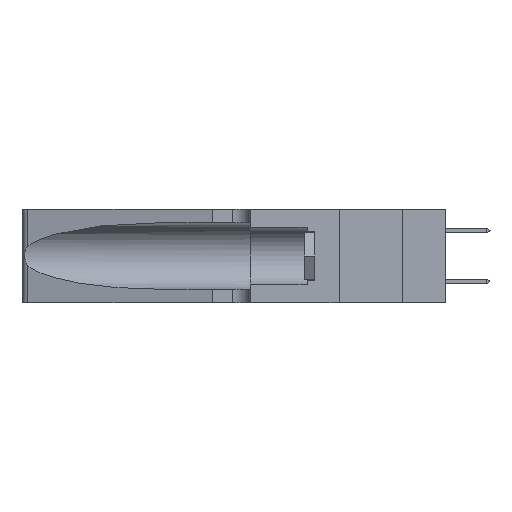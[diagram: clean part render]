
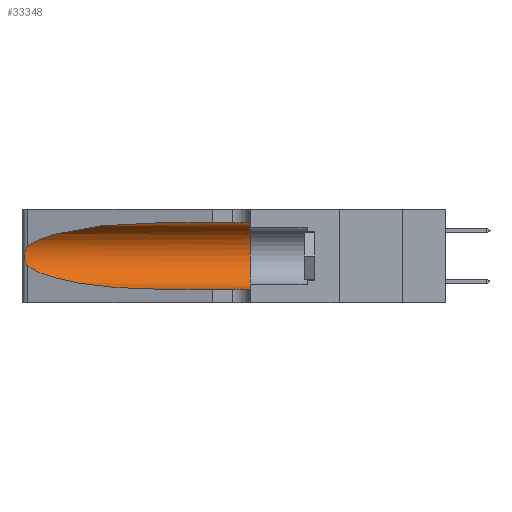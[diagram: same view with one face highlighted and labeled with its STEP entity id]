
A CAD part, left-side view. The second image highlights one B-rep face of the part: STEP entity #33348.
In plain terms, the highlighted cylindrical face has radius 3.308 mm (diameter 6.617 mm), a partial arc.
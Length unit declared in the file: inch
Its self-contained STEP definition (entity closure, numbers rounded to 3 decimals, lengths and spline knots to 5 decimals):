
#203 = FACE_OUTER_BOUND ( 'NONE', #29813, .T. ) ;
#289 = VECTOR ( 'NONE', #3742, 39.37008 ) ;
#589 = CARTESIAN_POINT ( 'NONE',  ( 0.25639, 1.23186, 0.15144 ) ) ;
#987 = EDGE_CURVE ( 'NONE', #16586, #30965, #5221, .T. ) ;
#1922 =( BOUNDED_CURVE ( )  B_SPLINE_CURVE ( 3, ( #33452, #4341, #13200, #30527 ),
 .UNSPECIFIED., .F., .F. ) 
 B_SPLINE_CURVE_WITH_KNOTS ( ( 4, 4 ),
 ( 1.5708, 2.84003 ),
 .UNSPECIFIED. ) 
 CURVE ( )  GEOMETRIC_REPRESENTATION_ITEM ( )  RATIONAL_B_SPLINE_CURVE ( ( 1., 0.87, 0.87, 1. ) ) 
 REPRESENTATION_ITEM ( '' )  );
#2430 = CARTESIAN_POINT ( 'NONE',  ( 0.1305, 0.35, 0.31525 ) ) ;
#3742 = DIRECTION ( 'NONE',  ( 0., -1., 0. ) ) ;
#4259 = CARTESIAN_POINT ( 'NONE',  ( 0.25487, 1.22718, 0.14631 ) ) ;
#4341 = CARTESIAN_POINT ( 'NONE',  ( 0.18966, 0.96281, 0.31525 ) ) ;
#4634 = CARTESIAN_POINT ( 'NONE',  ( 0.18966, 0.96281, 0.05475 ) ) ;
#4980 = ORIENTED_EDGE ( 'NONE', *, *, #33149, .F. ) ;
#5221 =( BOUNDED_CURVE ( )  B_SPLINE_CURVE ( 3, ( #4259, #10405, #4634, #7182 ),
 .UNSPECIFIED., .F., .F. ) 
 B_SPLINE_CURVE_WITH_KNOTS ( ( 4, 4 ),
 ( 3.44316, 4.71239 ),
 .UNSPECIFIED. ) 
 CURVE ( )  GEOMETRIC_REPRESENTATION_ITEM ( )  RATIONAL_B_SPLINE_CURVE ( ( 1., 0.87, 0.87, 1. ) ) 
 REPRESENTATION_ITEM ( '' )  );
#5313 = CARTESIAN_POINT ( 'NONE',  ( 0.26017, 1.23833, 0.17102 ) ) ;
#6033 = ORIENTED_EDGE ( 'NONE', *, *, #12997, .T. ) ;
#6106 = ORIENTED_EDGE ( 'NONE', *, *, #20171, .T. ) ;
#6560 = DIRECTION ( 'NONE',  ( 0., -1., 0. ) ) ;
#7096 = CARTESIAN_POINT ( 'NONE',  ( 0.1305, 0.72297, 0.05475 ) ) ;
#7182 = CARTESIAN_POINT ( 'NONE',  ( 0.1305, 0.72297, 0.05475 ) ) ;
#7240 = ORIENTED_EDGE ( 'NONE', *, *, #13904, .T. ) ;
#7669 = AXIS2_PLACEMENT_3D ( 'NONE', #24238, #27334, #27189 ) ;
#8811 = CARTESIAN_POINT ( 'NONE',  ( 0.25487, 1.22718, 0.14631 ) ) ;
#10405 = CARTESIAN_POINT ( 'NONE',  ( 0.2373, 1.15595, 0.08982 ) ) ;
#12116 = VERTEX_POINT ( 'NONE', #20535 ) ;
#12997 = EDGE_CURVE ( 'NONE', #30965, #31684, #14983, .T. ) ;
#13200 = CARTESIAN_POINT ( 'NONE',  ( 0.2373, 1.15595, 0.28018 ) ) ;
#13642 = ORIENTED_EDGE ( 'NONE', *, *, #987, .T. ) ;
#13904 = EDGE_CURVE ( 'NONE', #16901, #16586, #36481, .T. ) ;
#14732 = AXIS2_PLACEMENT_3D ( 'NONE', #30726, #30974, #19189 ) ;
#14983 = LINE ( 'NONE', #32971, #289 ) ;
#15815 = EDGE_CURVE ( 'NONE', #34322, #31684, #17096, .T. ) ;
#16586 = VERTEX_POINT ( 'NONE', #25327 ) ;
#16901 = VERTEX_POINT ( 'NONE', #21259 ) ;
#17096 = CIRCLE ( 'NONE', #7669, 0.13025 ) ;
#19189 = DIRECTION ( 'NONE',  ( 0., 0., -1. ) ) ;
#19609 = CARTESIAN_POINT ( 'NONE',  ( 0.25787, 1.23484, 0.2124 ) ) ;
#19867 = CARTESIAN_POINT ( 'NONE',  ( 0.26075, 1.23896, 0.178 ) ) ;
#19984 = CARTESIAN_POINT ( 'NONE',  ( 0.25639, 1.23184, 0.21858 ) ) ;
#20007 = LINE ( 'NONE', #21522, #21361 ) ;
#20171 = EDGE_CURVE ( 'NONE', #12116, #16901, #1922, .T. ) ;
#20535 = CARTESIAN_POINT ( 'NONE',  ( 0.1305, 0.72297, 0.31525 ) ) ;
#20667 = CARTESIAN_POINT ( 'NONE',  ( 0.25555, 1.22994, 0.2215 ) ) ;
#20928 = CYLINDRICAL_SURFACE ( 'NONE', #14732, 0.13025 ) ;
#21259 = CARTESIAN_POINT ( 'NONE',  ( 0.25487, 1.22718, 0.22369 ) ) ;
#21361 = VECTOR ( 'NONE', #6560, 39.37008 ) ;
#21522 = CARTESIAN_POINT ( 'NONE',  ( 0.1305, 1.61858, 0.31525 ) ) ;
#24238 = CARTESIAN_POINT ( 'NONE',  ( 0.1305, 0.35, 0.185 ) ) ;
#25327 = CARTESIAN_POINT ( 'NONE',  ( 0.25487, 1.22718, 0.14631 ) ) ;
#25488 = CARTESIAN_POINT ( 'NONE',  ( 0.1305, 0.35, 0.05475 ) ) ;
#26445 = CARTESIAN_POINT ( 'NONE',  ( 0.25487, 1.22718, 0.22369 ) ) ;
#27189 = DIRECTION ( 'NONE',  ( 0., 0., 1. ) ) ;
#27334 = DIRECTION ( 'NONE',  ( 0., 1., 0. ) ) ;
#29813 = EDGE_LOOP ( 'NONE', ( #6106, #7240, #13642, #6033, #30223, #4980 ) ) ;
#29897 = CARTESIAN_POINT ( 'NONE',  ( 0.25789, 1.23486, 0.15765 ) ) ;
#30223 = ORIENTED_EDGE ( 'NONE', *, *, #15815, .F. ) ;
#30527 = CARTESIAN_POINT ( 'NONE',  ( 0.25487, 1.22718, 0.22369 ) ) ;
#30726 = CARTESIAN_POINT ( 'NONE',  ( 0.1305, 1.61858, 0.185 ) ) ;
#30965 = VERTEX_POINT ( 'NONE', #7096 ) ;
#30974 = DIRECTION ( 'NONE',  ( 0., -1., 0. ) ) ;
#31384 = CARTESIAN_POINT ( 'NONE',  ( 0.25854, 1.2359, 0.20912 ) ) ;
#31507 = CARTESIAN_POINT ( 'NONE',  ( 0.25555, 1.22993, 0.14849 ) ) ;
#31684 = VERTEX_POINT ( 'NONE', #25488 ) ;
#32971 = CARTESIAN_POINT ( 'NONE',  ( 0.1305, 1.61858, 0.05475 ) ) ;
#33149 = EDGE_CURVE ( 'NONE', #12116, #34322, #20007, .T. ) ;
#33348 = ADVANCED_FACE ( 'NONE', ( #203 ), #20928, .F. ) ;
#33452 = CARTESIAN_POINT ( 'NONE',  ( 0.1305, 0.72297, 0.31525 ) ) ;
#34322 = VERTEX_POINT ( 'NONE', #2430 ) ;
#34330 = CARTESIAN_POINT ( 'NONE',  ( 0.26018, 1.23835, 0.19895 ) ) ;
#35494 = CARTESIAN_POINT ( 'NONE',  ( 0.25856, 1.23593, 0.16098 ) ) ;
#36481 = B_SPLINE_CURVE_WITH_KNOTS ( 'NONE', 3,
 ( #26445, #20667, #19984, #19609, #31384, #34330, #37388, #19867, #5313, #35494, #29897, #589, #31507, #8811 ),
 .UNSPECIFIED., .F., .F.,
 ( 4, 2, 2, 2, 2, 2, 4 ),
 ( 0., 0.00027, 0.00053, 0.00107, 0.0016, 0.00187, 0.00214 ),
 .UNSPECIFIED. ) ;
#37388 = CARTESIAN_POINT ( 'NONE',  ( 0.26075, 1.23896, 0.19203 ) ) ;
